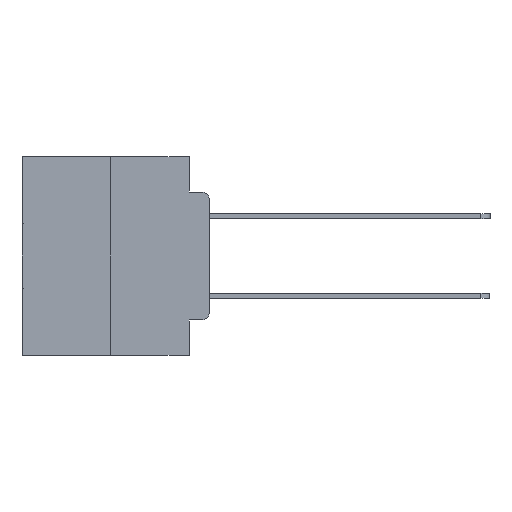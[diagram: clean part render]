
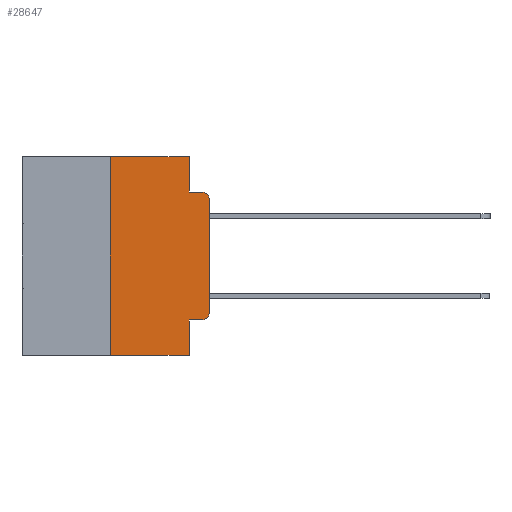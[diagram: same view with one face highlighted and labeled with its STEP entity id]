
A CAD part, left-side view. The second image highlights one B-rep face of the part: STEP entity #28647.
In plain terms, the highlighted planar face has unit normal (-1, 0, 0).
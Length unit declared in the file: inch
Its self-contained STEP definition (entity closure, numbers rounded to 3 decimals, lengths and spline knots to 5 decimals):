
#871 = ORIENTED_EDGE ( 'NONE', *, *, #17855, .F. ) ;
#874 = AXIS2_PLACEMENT_3D ( 'NONE', #2896, #18748, #5202 ) ;
#1480 = CARTESIAN_POINT ( 'NONE',  ( 0., 0.25, 0. ) ) ;
#1987 = PLANE ( 'NONE',  #8815 ) ;
#2334 = ORIENTED_EDGE ( 'NONE', *, *, #13140, .T. ) ;
#2642 = EDGE_CURVE ( 'NONE', #15509, #21294, #6280, .T. ) ;
#2896 = CARTESIAN_POINT ( 'NONE',  ( 0., 0.02, -0.1085 ) ) ;
#2963 = EDGE_LOOP ( 'NONE', ( #16168, #5566, #23614, #871, #13704, #25683, #2334, #15132, #27736, #17261 ) ) ;
#3640 = VERTEX_POINT ( 'NONE', #15401 ) ;
#5153 = EDGE_CURVE ( 'NONE', #23123, #19553, #18083, .T. ) ;
#5202 = DIRECTION ( 'NONE',  ( 0., 0., -1. ) ) ;
#5214 = CARTESIAN_POINT ( 'NONE',  ( 0., 0.02, -0.3915 ) ) ;
#5290 = VECTOR ( 'NONE', #27248, 39.37008 ) ;
#5566 = ORIENTED_EDGE ( 'NONE', *, *, #9792, .T. ) ;
#5912 = LINE ( 'NONE', #12193, #29072 ) ;
#5937 = VERTEX_POINT ( 'NONE', #25984 ) ;
#6280 = LINE ( 'NONE', #7123, #28741 ) ;
#6629 = DIRECTION ( 'NONE',  ( 1., 0., 0. ) ) ;
#7064 = CARTESIAN_POINT ( 'NONE',  ( 0., 0.473, -0.5 ) ) ;
#7123 = CARTESIAN_POINT ( 'NONE',  ( 0., 0.051, 0. ) ) ;
#7276 = EDGE_CURVE ( 'NONE', #23563, #7960, #26705, .T. ) ;
#7556 = DIRECTION ( 'NONE',  ( 0., 0., -1. ) ) ;
#7960 = VERTEX_POINT ( 'NONE', #15169 ) ;
#8185 = CARTESIAN_POINT ( 'NONE',  ( 0., 0.051, -0.4115 ) ) ;
#8215 = VECTOR ( 'NONE', #24779, 39.37008 ) ;
#8815 = AXIS2_PLACEMENT_3D ( 'NONE', #20138, #6629, #22412 ) ;
#9339 = CARTESIAN_POINT ( 'NONE',  ( 0., 0.051, -0.4115 ) ) ;
#9453 = CARTESIAN_POINT ( 'NONE',  ( 0., 0.02, -0.0885 ) ) ;
#9792 = EDGE_CURVE ( 'NONE', #22338, #19553, #26220, .T. ) ;
#10985 = EDGE_CURVE ( 'NONE', #7960, #3640, #5912, .T. ) ;
#12193 = CARTESIAN_POINT ( 'NONE',  ( 0., 0.473, 0. ) ) ;
#13140 = EDGE_CURVE ( 'NONE', #23563, #21294, #13919, .T. ) ;
#13147 = VERTEX_POINT ( 'NONE', #27293 ) ;
#13704 = ORIENTED_EDGE ( 'NONE', *, *, #10985, .F. ) ;
#13919 = LINE ( 'NONE', #7064, #18518 ) ;
#15103 = DIRECTION ( 'NONE',  ( 0., 0., 1. ) ) ;
#15132 = ORIENTED_EDGE ( 'NONE', *, *, #2642, .F. ) ;
#15169 = CARTESIAN_POINT ( 'NONE',  ( 0., 0.25, 0. ) ) ;
#15401 = CARTESIAN_POINT ( 'NONE',  ( 0., 0.051, 0. ) ) ;
#15509 = VERTEX_POINT ( 'NONE', #8185 ) ;
#15574 = LINE ( 'NONE', #22519, #8215 ) ;
#15772 = EDGE_CURVE ( 'NONE', #13147, #22338, #15574, .T. ) ;
#15940 = LINE ( 'NONE', #27646, #26488 ) ;
#15946 = CIRCLE ( 'NONE', #19069, 0.02 ) ;
#16168 = ORIENTED_EDGE ( 'NONE', *, *, #15772, .T. ) ;
#16491 = DIRECTION ( 'NONE',  ( 0., 0., -1. ) ) ;
#17261 = ORIENTED_EDGE ( 'NONE', *, *, #25540, .T. ) ;
#17855 = EDGE_CURVE ( 'NONE', #3640, #23123, #15940, .T. ) ;
#18083 = LINE ( 'NONE', #20649, #28535 ) ;
#18518 = VECTOR ( 'NONE', #20575, 39.37008 ) ;
#18636 = FACE_OUTER_BOUND ( 'NONE', #2963, .T. ) ;
#18748 = DIRECTION ( 'NONE',  ( -1., 0., 0. ) ) ;
#19069 = AXIS2_PLACEMENT_3D ( 'NONE', #5214, #21053, #7556 ) ;
#19553 = VERTEX_POINT ( 'NONE', #9453 ) ;
#20058 = VECTOR ( 'NONE', #15103, 39.37008 ) ;
#20138 = CARTESIAN_POINT ( 'NONE',  ( 0., 0.473, 0. ) ) ;
#20575 = DIRECTION ( 'NONE',  ( 0., -1., 0. ) ) ;
#20649 = CARTESIAN_POINT ( 'NONE',  ( 0., 0.051, -0.0885 ) ) ;
#21053 = DIRECTION ( 'NONE',  ( -1., 0., 0. ) ) ;
#21271 = DIRECTION ( 'NONE',  ( 0., -1., 0. ) ) ;
#21294 = VERTEX_POINT ( 'NONE', #24554 ) ;
#22338 = VERTEX_POINT ( 'NONE', #28526 ) ;
#22412 = DIRECTION ( 'NONE',  ( 0., 0., -1. ) ) ;
#22519 = CARTESIAN_POINT ( 'NONE',  ( 0., 0., 0. ) ) ;
#22910 = DIRECTION ( 'NONE',  ( 0., -1., 0. ) ) ;
#23123 = VERTEX_POINT ( 'NONE', #28958 ) ;
#23563 = VERTEX_POINT ( 'NONE', #28082 ) ;
#23614 = ORIENTED_EDGE ( 'NONE', *, *, #5153, .F. ) ;
#24554 = CARTESIAN_POINT ( 'NONE',  ( 0., 0.051, -0.5 ) ) ;
#24779 = DIRECTION ( 'NONE',  ( 0., 0., 1. ) ) ;
#25540 = EDGE_CURVE ( 'NONE', #5937, #13147, #15946, .T. ) ;
#25683 = ORIENTED_EDGE ( 'NONE', *, *, #7276, .F. ) ;
#25841 = DIRECTION ( 'NONE',  ( 0., 0., -1. ) ) ;
#25984 = CARTESIAN_POINT ( 'NONE',  ( 0., 0.02, -0.4115 ) ) ;
#26220 = CIRCLE ( 'NONE', #874, 0.02 ) ;
#26488 = VECTOR ( 'NONE', #16491, 39.37008 ) ;
#26705 = LINE ( 'NONE', #1480, #20058 ) ;
#27006 = EDGE_CURVE ( 'NONE', #15509, #5937, #28491, .T. ) ;
#27248 = DIRECTION ( 'NONE',  ( 0., -1., 0. ) ) ;
#27293 = CARTESIAN_POINT ( 'NONE',  ( 0., 0., -0.3915 ) ) ;
#27646 = CARTESIAN_POINT ( 'NONE',  ( 0., 0.051, 0. ) ) ;
#27736 = ORIENTED_EDGE ( 'NONE', *, *, #27006, .T. ) ;
#28082 = CARTESIAN_POINT ( 'NONE',  ( 0., 0.25, -0.5 ) ) ;
#28491 = LINE ( 'NONE', #9339, #5290 ) ;
#28526 = CARTESIAN_POINT ( 'NONE',  ( 0., 0., -0.1085 ) ) ;
#28535 = VECTOR ( 'NONE', #22910, 39.37008 ) ;
#28647 = ADVANCED_FACE ( 'NONE', ( #18636 ), #1987, .F. ) ;
#28741 = VECTOR ( 'NONE', #25841, 39.37008 ) ;
#28958 = CARTESIAN_POINT ( 'NONE',  ( 0., 0.051, -0.0885 ) ) ;
#29072 = VECTOR ( 'NONE', #21271, 39.37008 ) ;
